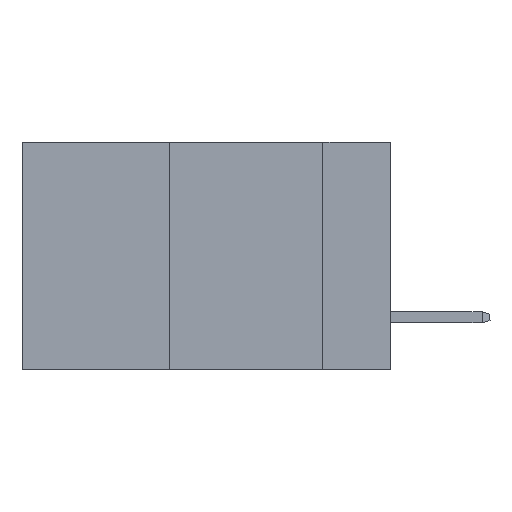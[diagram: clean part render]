
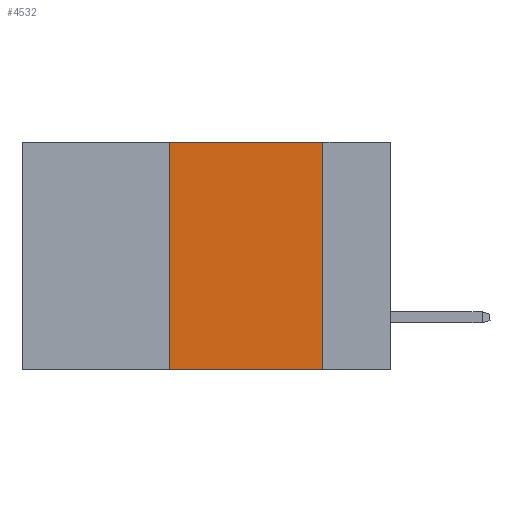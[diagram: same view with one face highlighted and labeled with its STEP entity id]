
A CAD part, left-side view. The second image highlights one B-rep face of the part: STEP entity #4532.
In plain terms, the highlighted planar face has unit normal (-1, 0, 0).
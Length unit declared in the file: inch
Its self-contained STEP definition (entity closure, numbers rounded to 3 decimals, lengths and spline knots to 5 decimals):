
#486 = ORIENTED_EDGE ( 'NONE', *, *, #2627, .F. ) ;
#535 = EDGE_CURVE ( 'NONE', #18355, #1148, #11451, .T. ) ;
#1148 = VERTEX_POINT ( 'NONE', #14530 ) ;
#1955 = VECTOR ( 'NONE', #20281, 39.37008 ) ;
#2100 = AXIS2_PLACEMENT_3D ( 'NONE', #21010, #10723, #25153 ) ;
#2178 = LINE ( 'NONE', #12514, #23545 ) ;
#2447 = ORIENTED_EDGE ( 'NONE', *, *, #535, .F. ) ;
#2627 = EDGE_CURVE ( 'NONE', #14649, #18355, #17127, .T. ) ;
#3823 = CARTESIAN_POINT ( 'NONE',  ( 0., 0.36, 0. ) ) ;
#4532 = ADVANCED_FACE ( 'NONE', ( #16060 ), #6556, .F. ) ;
#5098 = EDGE_LOOP ( 'NONE', ( #2447, #486, #12895, #12571 ) ) ;
#6315 = CARTESIAN_POINT ( 'NONE',  ( 0., 0.11, 0. ) ) ;
#6342 = DIRECTION ( 'NONE',  ( 0., -1., 0. ) ) ;
#6556 = PLANE ( 'NONE',  #2100 ) ;
#8260 = CARTESIAN_POINT ( 'NONE',  ( 0., 0.11, 0. ) ) ;
#9693 = VECTOR ( 'NONE', #13210, 39.37008 ) ;
#10679 = VERTEX_POINT ( 'NONE', #18082 ) ;
#10723 = DIRECTION ( 'NONE',  ( 1., 0., 0. ) ) ;
#11451 = LINE ( 'NONE', #8260, #16939 ) ;
#12514 = CARTESIAN_POINT ( 'NONE',  ( 0., 0.6, -0.37 ) ) ;
#12544 = DIRECTION ( 'NONE',  ( 0., 0., -1. ) ) ;
#12571 = ORIENTED_EDGE ( 'NONE', *, *, #22867, .T. ) ;
#12895 = ORIENTED_EDGE ( 'NONE', *, *, #20308, .F. ) ;
#13210 = DIRECTION ( 'NONE',  ( 0., -1., 0. ) ) ;
#14530 = CARTESIAN_POINT ( 'NONE',  ( 0., 0.11, -0.37 ) ) ;
#14649 = VERTEX_POINT ( 'NONE', #20993 ) ;
#16060 = FACE_OUTER_BOUND ( 'NONE', #5098, .T. ) ;
#16939 = VECTOR ( 'NONE', #12544, 39.37008 ) ;
#17127 = LINE ( 'NONE', #23438, #9693 ) ;
#17871 = LINE ( 'NONE', #3823, #1955 ) ;
#18082 = CARTESIAN_POINT ( 'NONE',  ( 0., 0.36, -0.37 ) ) ;
#18355 = VERTEX_POINT ( 'NONE', #6315 ) ;
#20281 = DIRECTION ( 'NONE',  ( 0., 0., 1. ) ) ;
#20308 = EDGE_CURVE ( 'NONE', #10679, #14649, #17871, .T. ) ;
#20993 = CARTESIAN_POINT ( 'NONE',  ( 0., 0.36, 0. ) ) ;
#21010 = CARTESIAN_POINT ( 'NONE',  ( 0., 0.6, 0. ) ) ;
#22867 = EDGE_CURVE ( 'NONE', #10679, #1148, #2178, .T. ) ;
#23438 = CARTESIAN_POINT ( 'NONE',  ( 0., 0.6, 0. ) ) ;
#23545 = VECTOR ( 'NONE', #6342, 39.37008 ) ;
#25153 = DIRECTION ( 'NONE',  ( 0., 0., -1. ) ) ;
